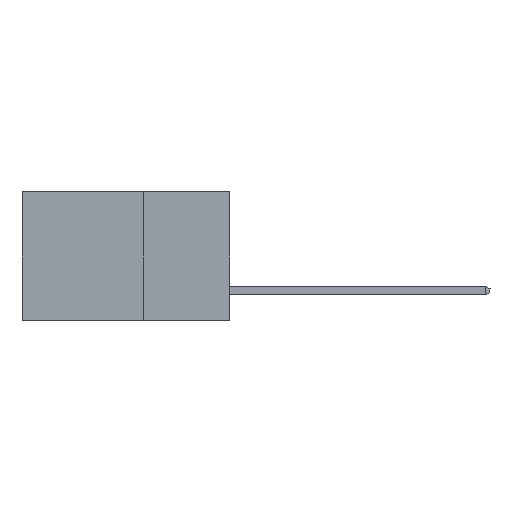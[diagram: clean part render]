
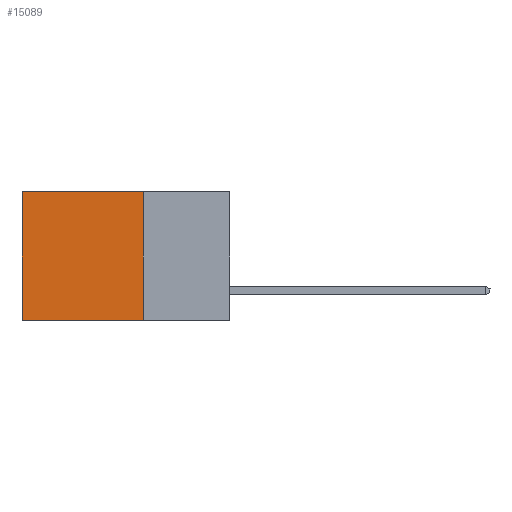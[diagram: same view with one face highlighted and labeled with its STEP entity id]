
A CAD part, left-side view. The second image highlights one B-rep face of the part: STEP entity #15089.
In plain terms, the highlighted planar face has unit normal (-1, 0, 0).
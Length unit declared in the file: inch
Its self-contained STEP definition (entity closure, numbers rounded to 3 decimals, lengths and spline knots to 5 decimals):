
#312 = LINE ( 'NONE', #3560, #11080 ) ;
#478 = CARTESIAN_POINT ( 'NONE',  ( 0.2615, 0.6, 0. ) ) ;
#1391 = CARTESIAN_POINT ( 'NONE',  ( 0.2615, 0.6, -0.37 ) ) ;
#1468 = DIRECTION ( 'NONE',  ( 0., 0., -1. ) ) ;
#1615 = EDGE_CURVE ( 'NONE', #5712, #9194, #312, .T. ) ;
#1829 = EDGE_CURVE ( 'NONE', #11667, #16952, #12320, .T. ) ;
#3256 = VECTOR ( 'NONE', #3506, 39.37008 ) ;
#3506 = DIRECTION ( 'NONE',  ( 0., 0., -1. ) ) ;
#3560 = CARTESIAN_POINT ( 'NONE',  ( 0.2615, 0.25, 0. ) ) ;
#4176 = LINE ( 'NONE', #9591, #9684 ) ;
#4341 = AXIS2_PLACEMENT_3D ( 'NONE', #9714, #17495, #1468 ) ;
#4831 = CARTESIAN_POINT ( 'NONE',  ( 0.2615, 0.6, -0.37 ) ) ;
#5712 = VERTEX_POINT ( 'NONE', #16941 ) ;
#6197 = ORIENTED_EDGE ( 'NONE', *, *, #1829, .F. ) ;
#6708 = ORIENTED_EDGE ( 'NONE', *, *, #10852, .F. ) ;
#6822 = ORIENTED_EDGE ( 'NONE', *, *, #1615, .T. ) ;
#6832 = CARTESIAN_POINT ( 'NONE',  ( 0.2615, 0.25, -0.37 ) ) ;
#7520 = ORIENTED_EDGE ( 'NONE', *, *, #17002, .T. ) ;
#8152 = EDGE_LOOP ( 'NONE', ( #7520, #6197, #6708, #6822 ) ) ;
#9194 = VERTEX_POINT ( 'NONE', #478 ) ;
#9591 = CARTESIAN_POINT ( 'NONE',  ( 0.2615, 0.25, -0.37 ) ) ;
#9684 = VECTOR ( 'NONE', #13645, 39.37008 ) ;
#9714 = CARTESIAN_POINT ( 'NONE',  ( 0.2615, 0.25, -0.37 ) ) ;
#9901 = LINE ( 'NONE', #4831, #3256 ) ;
#10852 = EDGE_CURVE ( 'NONE', #5712, #11667, #4176, .T. ) ;
#11080 = VECTOR ( 'NONE', #12532, 39.37008 ) ;
#11667 = VERTEX_POINT ( 'NONE', #17194 ) ;
#11939 = VECTOR ( 'NONE', #12408, 39.37008 ) ;
#12009 = FACE_OUTER_BOUND ( 'NONE', #8152, .T. ) ;
#12320 = LINE ( 'NONE', #6832, #11939 ) ;
#12408 = DIRECTION ( 'NONE',  ( 0., 1., 0. ) ) ;
#12532 = DIRECTION ( 'NONE',  ( 0., 1., 0. ) ) ;
#13645 = DIRECTION ( 'NONE',  ( 0., 0., -1. ) ) ;
#15089 = ADVANCED_FACE ( 'NONE', ( #12009 ), #17414, .F. ) ;
#16941 = CARTESIAN_POINT ( 'NONE',  ( 0.2615, 0.25, 0. ) ) ;
#16952 = VERTEX_POINT ( 'NONE', #1391 ) ;
#17002 = EDGE_CURVE ( 'NONE', #9194, #16952, #9901, .T. ) ;
#17194 = CARTESIAN_POINT ( 'NONE',  ( 0.2615, 0.25, -0.37 ) ) ;
#17414 = PLANE ( 'NONE',  #4341 ) ;
#17495 = DIRECTION ( 'NONE',  ( 1., 0., 0. ) ) ;
